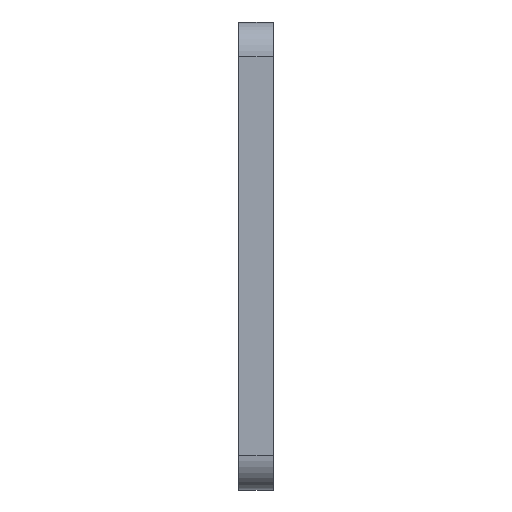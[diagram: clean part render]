
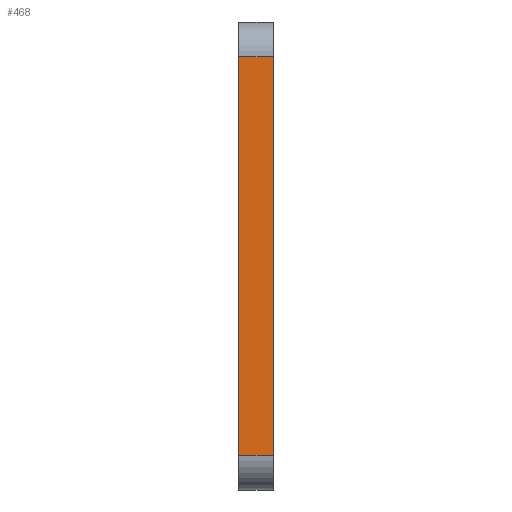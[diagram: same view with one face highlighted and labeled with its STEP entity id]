
A CAD part, left-side view. The second image highlights one B-rep face of the part: STEP entity #468.
In plain terms, the highlighted planar face has unit normal (-1, 0, 0).
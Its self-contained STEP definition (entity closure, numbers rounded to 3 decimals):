
#49 = FACE_OUTER_BOUND ( 'NONE', #180, .T. ) ;
#120 = VERTEX_POINT ( 'NONE', #1161 ) ;
#180 = EDGE_LOOP ( 'NONE', ( #432, #1130, #1118, #1451 ) ) ;
#195 = VECTOR ( 'NONE', #1197, 1000. ) ;
#221 = VECTOR ( 'NONE', #766, 1000. ) ;
#227 = VERTEX_POINT ( 'NONE', #1414 ) ;
#373 = DIRECTION ( 'NONE',  ( 0., 0., -1. ) ) ;
#432 = ORIENTED_EDGE ( 'NONE', *, *, #590, .T. ) ;
#468 = ADVANCED_FACE ( 'NONE', ( #49 ), #836, .F. ) ;
#480 = CARTESIAN_POINT ( 'NONE',  ( 0., 0., 16.15 ) ) ;
#535 = EDGE_CURVE ( 'NONE', #120, #227, #1079, .T. ) ;
#583 = EDGE_CURVE ( 'NONE', #120, #899, #845, .T. ) ;
#589 = VECTOR ( 'NONE', #1312, 1000. ) ;
#590 = EDGE_CURVE ( 'NONE', #227, #1360, #1306, .T. ) ;
#612 = CARTESIAN_POINT ( 'NONE',  ( 0., 1.3, 1.3 ) ) ;
#627 = DIRECTION ( 'NONE',  ( 1., 0., 0. ) ) ;
#674 = CARTESIAN_POINT ( 'NONE',  ( 0., 1.3, 16.15 ) ) ;
#684 = EDGE_CURVE ( 'NONE', #899, #1360, #1458, .T. ) ;
#766 = DIRECTION ( 'NONE',  ( 0., -1., 0. ) ) ;
#821 = CARTESIAN_POINT ( 'NONE',  ( 0., 1.3, 16.15 ) ) ;
#836 = PLANE ( 'NONE',  #1499 ) ;
#845 = LINE ( 'NONE', #821, #589 ) ;
#899 = VERTEX_POINT ( 'NONE', #674 ) ;
#944 = DIRECTION ( 'NONE',  ( 0., -1., 0. ) ) ;
#1001 = CARTESIAN_POINT ( 'NONE',  ( 0., 1.3, 16.15 ) ) ;
#1079 = LINE ( 'NONE', #612, #1419 ) ;
#1092 = CARTESIAN_POINT ( 'NONE',  ( 0., 1.3, 16.15 ) ) ;
#1118 = ORIENTED_EDGE ( 'NONE', *, *, #583, .F. ) ;
#1130 = ORIENTED_EDGE ( 'NONE', *, *, #684, .F. ) ;
#1161 = CARTESIAN_POINT ( 'NONE',  ( 0., 1.3, 1.3 ) ) ;
#1197 = DIRECTION ( 'NONE',  ( 0., 0., 1. ) ) ;
#1286 = CARTESIAN_POINT ( 'NONE',  ( 0., 0., 16.15 ) ) ;
#1306 = LINE ( 'NONE', #480, #195 ) ;
#1312 = DIRECTION ( 'NONE',  ( 0., 0., 1. ) ) ;
#1360 = VERTEX_POINT ( 'NONE', #1286 ) ;
#1414 = CARTESIAN_POINT ( 'NONE',  ( 0., 0., 1.3 ) ) ;
#1419 = VECTOR ( 'NONE', #944, 1000. ) ;
#1451 = ORIENTED_EDGE ( 'NONE', *, *, #535, .T. ) ;
#1458 = LINE ( 'NONE', #1001, #221 ) ;
#1499 = AXIS2_PLACEMENT_3D ( 'NONE', #1092, #627, #373 ) ;
